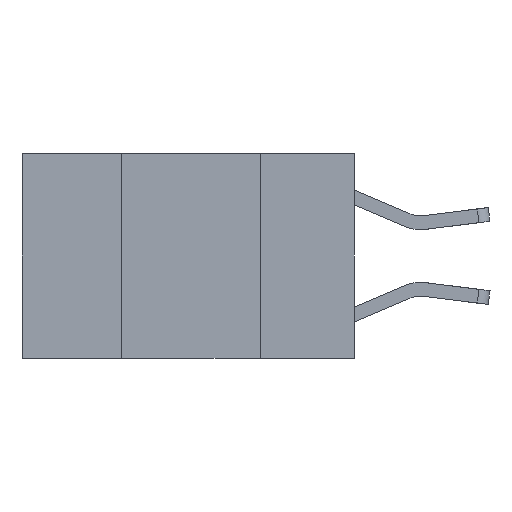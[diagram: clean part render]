
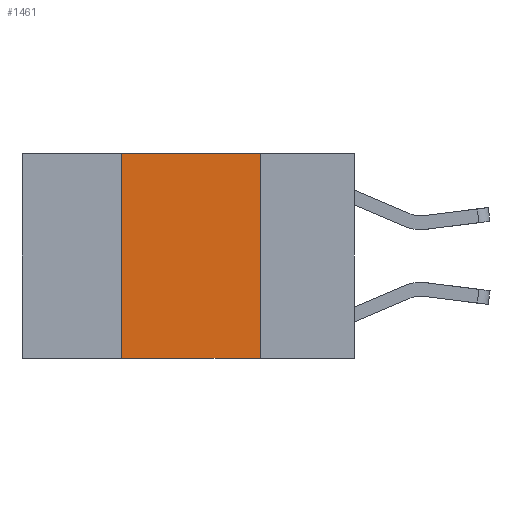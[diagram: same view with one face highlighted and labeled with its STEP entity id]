
A CAD part, left-side view. The second image highlights one B-rep face of the part: STEP entity #1461.
In plain terms, the highlighted planar face has unit normal (-1, 0, 0).
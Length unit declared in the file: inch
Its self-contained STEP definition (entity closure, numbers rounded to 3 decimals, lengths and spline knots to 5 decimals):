
#335 = CARTESIAN_POINT ( 'NONE',  ( 0., 0.6, -0.37 ) ) ;
#617 = LINE ( 'NONE', #335, #8954 ) ;
#1031 = EDGE_LOOP ( 'NONE', ( #10562, #7094, #3220, #3496 ) ) ;
#1048 = VERTEX_POINT ( 'NONE', #9468 ) ;
#1461 = ADVANCED_FACE ( 'NONE', ( #9976 ), #9845, .F. ) ;
#2628 = CARTESIAN_POINT ( 'NONE',  ( 0., 0.17, 0. ) ) ;
#2832 = VECTOR ( 'NONE', #6109, 39.37008 ) ;
#3208 = VECTOR ( 'NONE', #9420, 39.37008 ) ;
#3220 = ORIENTED_EDGE ( 'NONE', *, *, #9312, .F. ) ;
#3496 = ORIENTED_EDGE ( 'NONE', *, *, #7468, .T. ) ;
#3929 = AXIS2_PLACEMENT_3D ( 'NONE', #10033, #9731, #9694 ) ;
#4064 = CARTESIAN_POINT ( 'NONE',  ( 0., 0.42, -0.37 ) ) ;
#4703 = DIRECTION ( 'NONE',  ( 0., 0., 1. ) ) ;
#5161 = VECTOR ( 'NONE', #4703, 39.37008 ) ;
#5290 = LINE ( 'NONE', #8505, #2832 ) ;
#6109 = DIRECTION ( 'NONE',  ( 0., 0., -1. ) ) ;
#6387 = VERTEX_POINT ( 'NONE', #2628 ) ;
#6875 = VERTEX_POINT ( 'NONE', #4064 ) ;
#7014 = CARTESIAN_POINT ( 'NONE',  ( 0., 0.42, 0. ) ) ;
#7094 = ORIENTED_EDGE ( 'NONE', *, *, #7395, .F. ) ;
#7323 = LINE ( 'NONE', #7919, #5161 ) ;
#7395 = EDGE_CURVE ( 'NONE', #9960, #6387, #9682, .T. ) ;
#7468 = EDGE_CURVE ( 'NONE', #6875, #1048, #617, .T. ) ;
#7827 = CARTESIAN_POINT ( 'NONE',  ( 0., 0.6, 0. ) ) ;
#7919 = CARTESIAN_POINT ( 'NONE',  ( 0., 0.42, 0. ) ) ;
#8505 = CARTESIAN_POINT ( 'NONE',  ( 0., 0.17, 0. ) ) ;
#8723 = DIRECTION ( 'NONE',  ( 0., -1., 0. ) ) ;
#8954 = VECTOR ( 'NONE', #8723, 39.37008 ) ;
#9099 = EDGE_CURVE ( 'NONE', #6387, #1048, #5290, .T. ) ;
#9312 = EDGE_CURVE ( 'NONE', #6875, #9960, #7323, .T. ) ;
#9420 = DIRECTION ( 'NONE',  ( 0., -1., 0. ) ) ;
#9468 = CARTESIAN_POINT ( 'NONE',  ( 0., 0.17, -0.37 ) ) ;
#9682 = LINE ( 'NONE', #7827, #3208 ) ;
#9694 = DIRECTION ( 'NONE',  ( 0., 0., -1. ) ) ;
#9731 = DIRECTION ( 'NONE',  ( 1., 0., 0. ) ) ;
#9845 = PLANE ( 'NONE',  #3929 ) ;
#9960 = VERTEX_POINT ( 'NONE', #7014 ) ;
#9976 = FACE_OUTER_BOUND ( 'NONE', #1031, .T. ) ;
#10033 = CARTESIAN_POINT ( 'NONE',  ( 0., 0.6, 0. ) ) ;
#10562 = ORIENTED_EDGE ( 'NONE', *, *, #9099, .F. ) ;
